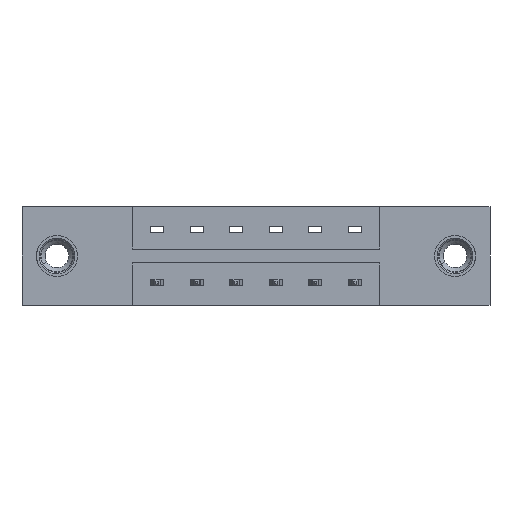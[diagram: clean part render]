
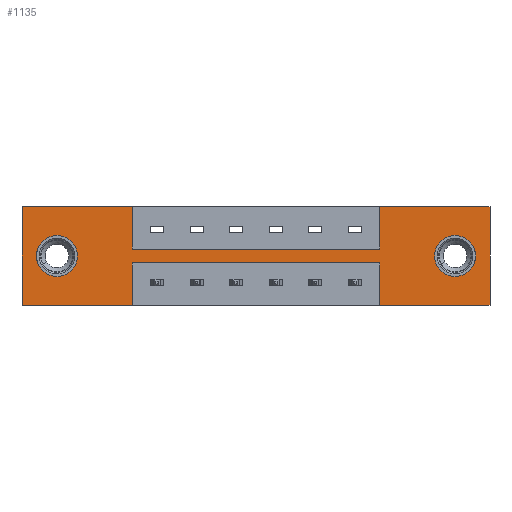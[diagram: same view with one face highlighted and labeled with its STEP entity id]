
A CAD part, front view. The second image highlights one B-rep face of the part: STEP entity #1135.
In plain terms, the highlighted planar face has unit normal (0, -1, 0).
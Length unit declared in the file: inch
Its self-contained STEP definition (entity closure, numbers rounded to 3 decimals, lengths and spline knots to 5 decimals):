
#92 = ORIENTED_EDGE ( 'NONE', *, *, #2175, .F. ) ;
#138 = CARTESIAN_POINT ( 'NONE',  ( 0., 0., -0.375 ) ) ;
#276 = CARTESIAN_POINT ( 'NONE',  ( 0., 0., -0.375 ) ) ;
#392 = DIRECTION ( 'NONE',  ( 0., 0., 1. ) ) ;
#418 = DIRECTION ( 'NONE',  ( 0., 0., -1. ) ) ;
#538 = CARTESIAN_POINT ( 'NONE',  ( 0., 0., -0.375 ) ) ;
#581 = VERTEX_POINT ( 'NONE', #4005 ) ;
#610 = EDGE_CURVE ( 'NONE', #6206, #6213, #2379, .T. ) ;
#643 = CARTESIAN_POINT ( 'NONE',  ( 1.3575, 0., -0.214 ) ) ;
#647 = DIRECTION ( 'NONE',  ( 1., 0., 0. ) ) ;
#782 = EDGE_CURVE ( 'NONE', #6213, #1309, #7989, .T. ) ;
#825 = PLANE ( 'NONE',  #9218 ) ;
#858 = LINE ( 'NONE', #4038, #9257 ) ;
#874 = CARTESIAN_POINT ( 'NONE',  ( 0.1325, 0., -0.1095 ) ) ;
#1007 = DIRECTION ( 'NONE',  ( 1., 0., 0. ) ) ;
#1042 = ORIENTED_EDGE ( 'NONE', *, *, #8809, .F. ) ;
#1102 = CARTESIAN_POINT ( 'NONE',  ( 0.4175, 0., -0.161 ) ) ;
#1115 = VERTEX_POINT ( 'NONE', #3723 ) ;
#1135 = ADVANCED_FACE ( 'NONE', ( #5220, #9126, #7625 ), #825, .T. ) ;
#1309 = VERTEX_POINT ( 'NONE', #3234 ) ;
#1428 = VERTEX_POINT ( 'NONE', #1875 ) ;
#1466 = EDGE_CURVE ( 'NONE', #1115, #4996, #5784, .T. ) ;
#1511 = ORIENTED_EDGE ( 'NONE', *, *, #2590, .T. ) ;
#1544 = VERTEX_POINT ( 'NONE', #7188 ) ;
#1561 = ORIENTED_EDGE ( 'NONE', *, *, #6427, .F. ) ;
#1573 = CIRCLE ( 'NONE', #7905, 0.078 ) ;
#1638 = ORIENTED_EDGE ( 'NONE', *, *, #610, .F. ) ;
#1699 = LINE ( 'NONE', #276, #9497 ) ;
#1708 = CARTESIAN_POINT ( 'NONE',  ( 0., 0., 0. ) ) ;
#1739 = ORIENTED_EDGE ( 'NONE', *, *, #6032, .F. ) ;
#1745 = DIRECTION ( 'NONE',  ( 0., 0., 1. ) ) ;
#1816 = DIRECTION ( 'NONE',  ( -1., 0., 0. ) ) ;
#1875 = CARTESIAN_POINT ( 'NONE',  ( 0., 0., 0. ) ) ;
#1971 = DIRECTION ( 'NONE',  ( 0., 0., 1. ) ) ;
#2015 = DIRECTION ( 'NONE',  ( 0., 0., 1. ) ) ;
#2175 = EDGE_CURVE ( 'NONE', #7525, #1115, #7026, .T. ) ;
#2273 = VERTEX_POINT ( 'NONE', #4337 ) ;
#2379 = LINE ( 'NONE', #3979, #4077 ) ;
#2577 = VERTEX_POINT ( 'NONE', #8584 ) ;
#2590 = EDGE_CURVE ( 'NONE', #4963, #3911, #8526, .T. ) ;
#2778 = DIRECTION ( 'NONE',  ( 0., 1., 0. ) ) ;
#2822 = CARTESIAN_POINT ( 'NONE',  ( 0., 0., 0. ) ) ;
#3020 = CARTESIAN_POINT ( 'NONE',  ( 1.6425, 0., -0.1875 ) ) ;
#3234 = CARTESIAN_POINT ( 'NONE',  ( 0.4175, 0., -0.375 ) ) ;
#3304 = CARTESIAN_POINT ( 'NONE',  ( 0.4175, 0., -0.214 ) ) ;
#3381 = EDGE_LOOP ( 'NONE', ( #1561, #1042, #4298, #92, #6698, #6913, #4780, #1739, #6021, #8762, #4781, #1638 ) ) ;
#3464 = AXIS2_PLACEMENT_3D ( 'NONE', #3020, #8131, #4483 ) ;
#3471 = CARTESIAN_POINT ( 'NONE',  ( 0.1325, 0., -0.1875 ) ) ;
#3625 = VECTOR ( 'NONE', #1745, 39.37008 ) ;
#3696 = VECTOR ( 'NONE', #647, 39.37008 ) ;
#3720 = CARTESIAN_POINT ( 'NONE',  ( 1.775, 0., -0.375 ) ) ;
#3723 = CARTESIAN_POINT ( 'NONE',  ( 1.775, 0., 0. ) ) ;
#3793 = LINE ( 'NONE', #4825, #9536 ) ;
#3842 = CARTESIAN_POINT ( 'NONE',  ( 0.4175, 0., -0.161 ) ) ;
#3911 = VERTEX_POINT ( 'NONE', #874 ) ;
#3918 = DIRECTION ( 'NONE',  ( -1., 0., 0. ) ) ;
#3926 = VECTOR ( 'NONE', #5390, 39.37008 ) ;
#3979 = CARTESIAN_POINT ( 'NONE',  ( 0.4175, 0., -0.214 ) ) ;
#4005 = CARTESIAN_POINT ( 'NONE',  ( 1.6425, 0., -0.2655 ) ) ;
#4038 = CARTESIAN_POINT ( 'NONE',  ( 1.3575, 0., -0.161 ) ) ;
#4077 = VECTOR ( 'NONE', #1816, 39.37008 ) ;
#4094 = CARTESIAN_POINT ( 'NONE',  ( 1.775, 0., 0. ) ) ;
#4177 = DIRECTION ( 'NONE',  ( 0., 1., 0. ) ) ;
#4194 = VECTOR ( 'NONE', #8230, 39.37008 ) ;
#4267 = DIRECTION ( 'NONE',  ( 0., 0., -1. ) ) ;
#4298 = ORIENTED_EDGE ( 'NONE', *, *, #1466, .F. ) ;
#4337 = CARTESIAN_POINT ( 'NONE',  ( 0.4175, 0., 0. ) ) ;
#4470 = LINE ( 'NONE', #8267, #7701 ) ;
#4483 = DIRECTION ( 'NONE',  ( 0., 0., -1. ) ) ;
#4550 = DIRECTION ( 'NONE',  ( 0., -1., 0. ) ) ;
#4604 = AXIS2_PLACEMENT_3D ( 'NONE', #3471, #4177, #2015 ) ;
#4643 = CARTESIAN_POINT ( 'NONE',  ( 1.3575, 0., 0. ) ) ;
#4780 = ORIENTED_EDGE ( 'NONE', *, *, #5212, .F. ) ;
#4781 = ORIENTED_EDGE ( 'NONE', *, *, #782, .F. ) ;
#4818 = DIRECTION ( 'NONE',  ( 0., 0., -1. ) ) ;
#4825 = CARTESIAN_POINT ( 'NONE',  ( 0., 0., 0. ) ) ;
#4963 = VERTEX_POINT ( 'NONE', #9400 ) ;
#4996 = VERTEX_POINT ( 'NONE', #3720 ) ;
#5010 = AXIS2_PLACEMENT_3D ( 'NONE', #6361, #9252, #1971 ) ;
#5212 = EDGE_CURVE ( 'NONE', #2273, #9481, #7261, .T. ) ;
#5220 = FACE_BOUND ( 'NONE', #5660, .T. ) ;
#5289 = EDGE_CURVE ( 'NONE', #9481, #9068, #9106, .T. ) ;
#5364 = CIRCLE ( 'NONE', #3464, 0.078 ) ;
#5390 = DIRECTION ( 'NONE',  ( 0., 0., -1. ) ) ;
#5446 = ORIENTED_EDGE ( 'NONE', *, *, #8463, .T. ) ;
#5660 = EDGE_LOOP ( 'NONE', ( #8818, #5446 ) ) ;
#5784 = LINE ( 'NONE', #4094, #7507 ) ;
#6021 = ORIENTED_EDGE ( 'NONE', *, *, #8970, .F. ) ;
#6032 = EDGE_CURVE ( 'NONE', #1428, #2273, #3793, .T. ) ;
#6074 = CIRCLE ( 'NONE', #5010, 0.078 ) ;
#6135 = VERTEX_POINT ( 'NONE', #538 ) ;
#6155 = LINE ( 'NONE', #138, #4194 ) ;
#6206 = VERTEX_POINT ( 'NONE', #643 ) ;
#6213 = VERTEX_POINT ( 'NONE', #9447 ) ;
#6361 = CARTESIAN_POINT ( 'NONE',  ( 0.1325, 0., -0.1875 ) ) ;
#6427 = EDGE_CURVE ( 'NONE', #1544, #6206, #4470, .T. ) ;
#6650 = DIRECTION ( 'NONE',  ( 0., 0., 1. ) ) ;
#6677 = CARTESIAN_POINT ( 'NONE',  ( 0., 0., -0.375 ) ) ;
#6698 = ORIENTED_EDGE ( 'NONE', *, *, #9159, .F. ) ;
#6913 = ORIENTED_EDGE ( 'NONE', *, *, #5289, .F. ) ;
#6956 = CARTESIAN_POINT ( 'NONE',  ( 0.4175, 0., -0.161 ) ) ;
#7026 = LINE ( 'NONE', #2822, #3696 ) ;
#7164 = EDGE_CURVE ( 'NONE', #3911, #4963, #6074, .T. ) ;
#7170 = CARTESIAN_POINT ( 'NONE',  ( 1.6425, 0., -0.1875 ) ) ;
#7188 = CARTESIAN_POINT ( 'NONE',  ( 1.3575, 0., -0.375 ) ) ;
#7261 = LINE ( 'NONE', #3842, #3926 ) ;
#7287 = ORIENTED_EDGE ( 'NONE', *, *, #7164, .T. ) ;
#7376 = VECTOR ( 'NONE', #1007, 39.37008 ) ;
#7415 = LINE ( 'NONE', #1708, #3625 ) ;
#7507 = VECTOR ( 'NONE', #418, 39.37008 ) ;
#7525 = VERTEX_POINT ( 'NONE', #4643 ) ;
#7625 = FACE_OUTER_BOUND ( 'NONE', #3381, .T. ) ;
#7701 = VECTOR ( 'NONE', #6650, 39.37008 ) ;
#7735 = CARTESIAN_POINT ( 'NONE',  ( 1.3575, 0., -0.161 ) ) ;
#7784 = DIRECTION ( 'NONE',  ( 1., 0., 0. ) ) ;
#7905 = AXIS2_PLACEMENT_3D ( 'NONE', #7170, #2778, #4267 ) ;
#7989 = LINE ( 'NONE', #3304, #8785 ) ;
#8131 = DIRECTION ( 'NONE',  ( 0., 1., 0. ) ) ;
#8230 = DIRECTION ( 'NONE',  ( -1., 0., 0. ) ) ;
#8251 = EDGE_CURVE ( 'NONE', #1309, #6135, #1699, .T. ) ;
#8267 = CARTESIAN_POINT ( 'NONE',  ( 1.3575, 0., -0.214 ) ) ;
#8463 = EDGE_CURVE ( 'NONE', #581, #2577, #1573, .T. ) ;
#8526 = CIRCLE ( 'NONE', #4604, 0.078 ) ;
#8584 = CARTESIAN_POINT ( 'NONE',  ( 1.6425, 0., -0.1095 ) ) ;
#8643 = EDGE_LOOP ( 'NONE', ( #7287, #1511 ) ) ;
#8762 = ORIENTED_EDGE ( 'NONE', *, *, #8251, .F. ) ;
#8769 = EDGE_CURVE ( 'NONE', #2577, #581, #5364, .T. ) ;
#8785 = VECTOR ( 'NONE', #4818, 39.37008 ) ;
#8809 = EDGE_CURVE ( 'NONE', #4996, #1544, #6155, .T. ) ;
#8818 = ORIENTED_EDGE ( 'NONE', *, *, #8769, .T. ) ;
#8861 = DIRECTION ( 'NONE',  ( 0., 0., -1. ) ) ;
#8970 = EDGE_CURVE ( 'NONE', #6135, #1428, #7415, .T. ) ;
#9068 = VERTEX_POINT ( 'NONE', #7735 ) ;
#9106 = LINE ( 'NONE', #6956, #7376 ) ;
#9126 = FACE_BOUND ( 'NONE', #8643, .T. ) ;
#9159 = EDGE_CURVE ( 'NONE', #9068, #7525, #858, .T. ) ;
#9218 = AXIS2_PLACEMENT_3D ( 'NONE', #6677, #4550, #8861 ) ;
#9252 = DIRECTION ( 'NONE',  ( 0., 1., 0. ) ) ;
#9257 = VECTOR ( 'NONE', #392, 39.37008 ) ;
#9400 = CARTESIAN_POINT ( 'NONE',  ( 0.1325, 0., -0.2655 ) ) ;
#9447 = CARTESIAN_POINT ( 'NONE',  ( 0.4175, 0., -0.214 ) ) ;
#9481 = VERTEX_POINT ( 'NONE', #1102 ) ;
#9497 = VECTOR ( 'NONE', #3918, 39.37008 ) ;
#9536 = VECTOR ( 'NONE', #7784, 39.37008 ) ;
